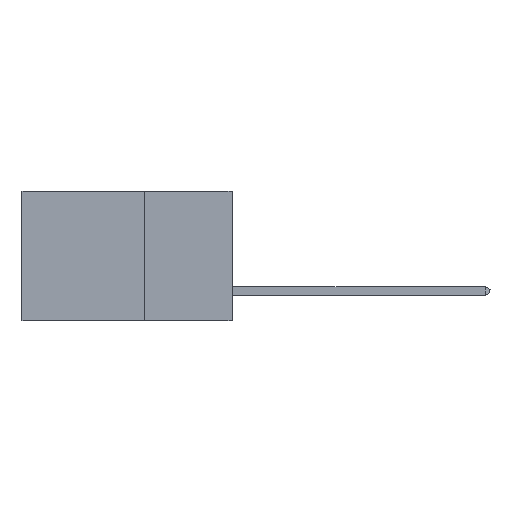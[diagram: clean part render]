
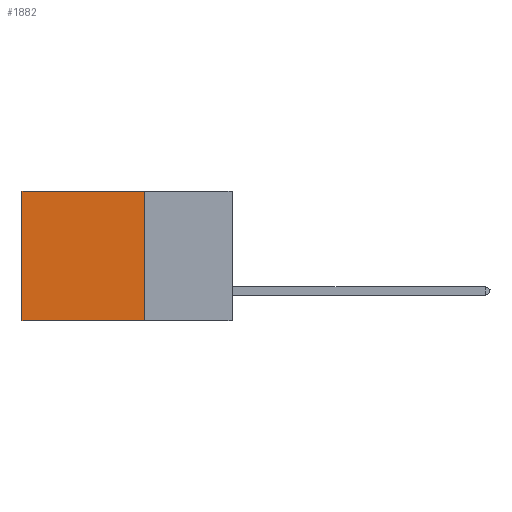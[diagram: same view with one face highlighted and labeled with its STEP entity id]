
A CAD part, left-side view. The second image highlights one B-rep face of the part: STEP entity #1882.
In plain terms, the highlighted planar face has unit normal (-1, 0, 0).
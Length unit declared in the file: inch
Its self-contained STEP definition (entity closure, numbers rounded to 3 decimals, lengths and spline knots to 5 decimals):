
#1442 = DIRECTION ( 'NONE',  ( 0., 0., -1. ) ) ;
#1882 = ADVANCED_FACE ( 'NONE', ( #44727 ), #27318, .F. ) ;
#2597 = AXIS2_PLACEMENT_3D ( 'NONE', #30790, #34233, #23567 ) ;
#3819 = CARTESIAN_POINT ( 'NONE',  ( 0.2875, 0.25, 0. ) ) ;
#4913 = CARTESIAN_POINT ( 'NONE',  ( 0.2875, 0.6, 0. ) ) ;
#6563 = EDGE_LOOP ( 'NONE', ( #28596, #42660, #7848, #7810 ) ) ;
#7233 = EDGE_CURVE ( 'NONE', #34377, #44082, #32130, .T. ) ;
#7810 = ORIENTED_EDGE ( 'NONE', *, *, #22095, .T. ) ;
#7848 = ORIENTED_EDGE ( 'NONE', *, *, #7233, .F. ) ;
#8077 = CARTESIAN_POINT ( 'NONE',  ( 0.2875, 0.25, -0.37 ) ) ;
#8093 = LINE ( 'NONE', #33257, #35443 ) ;
#10906 = VECTOR ( 'NONE', #36897, 39.37008 ) ;
#11862 = CARTESIAN_POINT ( 'NONE',  ( 0.2875, 0.25, 0. ) ) ;
#15882 = DIRECTION ( 'NONE',  ( 0., 1., 0. ) ) ;
#19833 = VECTOR ( 'NONE', #21833, 39.37008 ) ;
#21833 = DIRECTION ( 'NONE',  ( 0., 0., -1. ) ) ;
#22018 = LINE ( 'NONE', #22993, #10906 ) ;
#22095 = EDGE_CURVE ( 'NONE', #34377, #35490, #22018, .T. ) ;
#22993 = CARTESIAN_POINT ( 'NONE',  ( 0.2875, 0.25, 0. ) ) ;
#23567 = DIRECTION ( 'NONE',  ( 0., 0., -1. ) ) ;
#24331 = CARTESIAN_POINT ( 'NONE',  ( 0.2875, 0.6, -0.37 ) ) ;
#25897 = VERTEX_POINT ( 'NONE', #24331 ) ;
#27318 = PLANE ( 'NONE',  #2597 ) ;
#28596 = ORIENTED_EDGE ( 'NONE', *, *, #39048, .T. ) ;
#30790 = CARTESIAN_POINT ( 'NONE',  ( 0.2875, 0.25, 0. ) ) ;
#32130 = LINE ( 'NONE', #3819, #19833 ) ;
#33257 = CARTESIAN_POINT ( 'NONE',  ( 0.2875, 0.6, 0. ) ) ;
#33472 = LINE ( 'NONE', #44445, #41811 ) ;
#34233 = DIRECTION ( 'NONE',  ( 1., 0., 0. ) ) ;
#34377 = VERTEX_POINT ( 'NONE', #11862 ) ;
#35443 = VECTOR ( 'NONE', #1442, 39.37008 ) ;
#35490 = VERTEX_POINT ( 'NONE', #4913 ) ;
#36770 = EDGE_CURVE ( 'NONE', #44082, #25897, #33472, .T. ) ;
#36897 = DIRECTION ( 'NONE',  ( 0., 1., 0. ) ) ;
#39048 = EDGE_CURVE ( 'NONE', #35490, #25897, #8093, .T. ) ;
#41811 = VECTOR ( 'NONE', #15882, 39.37008 ) ;
#42660 = ORIENTED_EDGE ( 'NONE', *, *, #36770, .F. ) ;
#44082 = VERTEX_POINT ( 'NONE', #8077 ) ;
#44445 = CARTESIAN_POINT ( 'NONE',  ( 0.2875, 0.25, -0.37 ) ) ;
#44727 = FACE_OUTER_BOUND ( 'NONE', #6563, .T. ) ;
